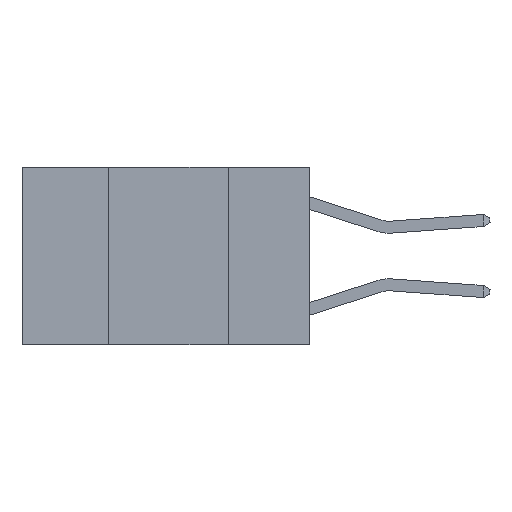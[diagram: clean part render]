
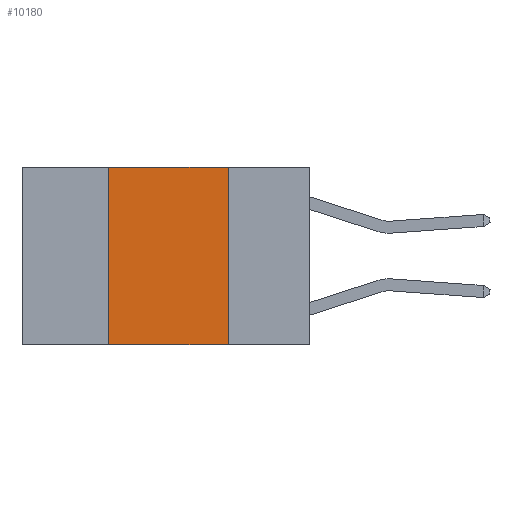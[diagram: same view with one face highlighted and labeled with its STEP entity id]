
A CAD part, left-side view. The second image highlights one B-rep face of the part: STEP entity #10180.
In plain terms, the highlighted planar face has unit normal (-1, 0, 0).
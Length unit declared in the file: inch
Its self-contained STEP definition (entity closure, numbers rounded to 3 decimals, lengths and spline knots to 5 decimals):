
#1323 = DIRECTION ( 'NONE',  ( 1., 0., 0. ) ) ;
#1732 = CARTESIAN_POINT ( 'NONE',  ( 0., 0.17, 0. ) ) ;
#2159 = AXIS2_PLACEMENT_3D ( 'NONE', #22020, #1323, #22134 ) ;
#2458 = LINE ( 'NONE', #7831, #13691 ) ;
#3315 = CARTESIAN_POINT ( 'NONE',  ( 0., 0.42, 0. ) ) ;
#3707 = CARTESIAN_POINT ( 'NONE',  ( 0., 0.6, 0. ) ) ;
#3968 = LINE ( 'NONE', #3707, #5172 ) ;
#3987 = LINE ( 'NONE', #11530, #13806 ) ;
#4523 = LINE ( 'NONE', #19810, #9922 ) ;
#5172 = VECTOR ( 'NONE', #9486, 39.37008 ) ;
#5490 = VERTEX_POINT ( 'NONE', #12524 ) ;
#7198 = VERTEX_POINT ( 'NONE', #1732 ) ;
#7325 = CARTESIAN_POINT ( 'NONE',  ( 0., 0.17, -0.37 ) ) ;
#7831 = CARTESIAN_POINT ( 'NONE',  ( 0., 0.17, 0. ) ) ;
#8758 = DIRECTION ( 'NONE',  ( 0., 0., 1. ) ) ;
#9486 = DIRECTION ( 'NONE',  ( 0., -1., 0. ) ) ;
#9779 = ORIENTED_EDGE ( 'NONE', *, *, #13242, .F. ) ;
#9922 = VECTOR ( 'NONE', #8758, 39.37008 ) ;
#10083 = DIRECTION ( 'NONE',  ( 0., 0., -1. ) ) ;
#10180 = ADVANCED_FACE ( 'NONE', ( #24011 ), #14682, .F. ) ;
#11530 = CARTESIAN_POINT ( 'NONE',  ( 0., 0.6, -0.37 ) ) ;
#12524 = CARTESIAN_POINT ( 'NONE',  ( 0., 0.42, -0.37 ) ) ;
#13242 = EDGE_CURVE ( 'NONE', #23907, #7198, #3968, .T. ) ;
#13691 = VECTOR ( 'NONE', #10083, 39.37008 ) ;
#13806 = VECTOR ( 'NONE', #18929, 39.37008 ) ;
#14122 = ORIENTED_EDGE ( 'NONE', *, *, #14505, .F. ) ;
#14505 = EDGE_CURVE ( 'NONE', #5490, #23907, #4523, .T. ) ;
#14682 = PLANE ( 'NONE',  #2159 ) ;
#15050 = EDGE_CURVE ( 'NONE', #7198, #15614, #2458, .T. ) ;
#15132 = ORIENTED_EDGE ( 'NONE', *, *, #15050, .F. ) ;
#15614 = VERTEX_POINT ( 'NONE', #7325 ) ;
#18929 = DIRECTION ( 'NONE',  ( 0., -1., 0. ) ) ;
#19810 = CARTESIAN_POINT ( 'NONE',  ( 0., 0.42, 0. ) ) ;
#21159 = EDGE_LOOP ( 'NONE', ( #15132, #9779, #14122, #23360 ) ) ;
#22020 = CARTESIAN_POINT ( 'NONE',  ( 0., 0.6, 0. ) ) ;
#22134 = DIRECTION ( 'NONE',  ( 0., 0., -1. ) ) ;
#22851 = EDGE_CURVE ( 'NONE', #5490, #15614, #3987, .T. ) ;
#23360 = ORIENTED_EDGE ( 'NONE', *, *, #22851, .T. ) ;
#23907 = VERTEX_POINT ( 'NONE', #3315 ) ;
#24011 = FACE_OUTER_BOUND ( 'NONE', #21159, .T. ) ;
